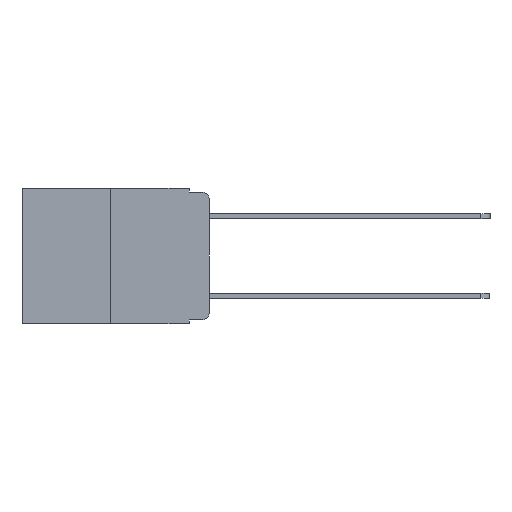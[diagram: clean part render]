
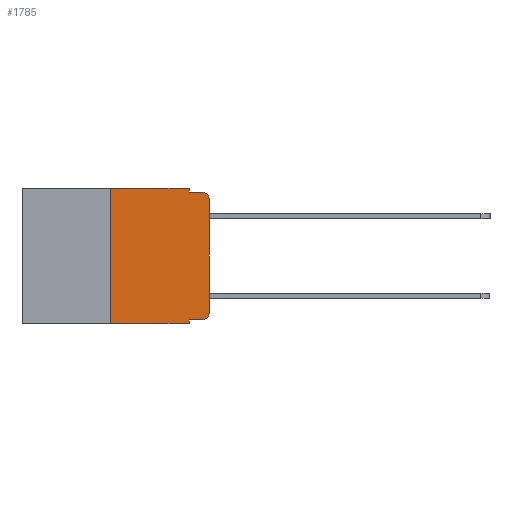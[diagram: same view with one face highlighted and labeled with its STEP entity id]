
A CAD part, left-side view. The second image highlights one B-rep face of the part: STEP entity #1785.
In plain terms, the highlighted planar face has unit normal (-1, 0, 0).
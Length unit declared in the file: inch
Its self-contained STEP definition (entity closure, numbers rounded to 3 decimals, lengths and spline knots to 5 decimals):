
#318 = LINE ( 'NONE', #8978, #4786 ) ;
#634 = DIRECTION ( 'NONE',  ( 0., 0., -1. ) ) ;
#671 = EDGE_CURVE ( 'NONE', #1986, #4047, #6278, .T. ) ;
#700 = ORIENTED_EDGE ( 'NONE', *, *, #8965, .T. ) ;
#863 = ORIENTED_EDGE ( 'NONE', *, *, #8610, .F. ) ;
#1166 = DIRECTION ( 'NONE',  ( 0., 0., 1. ) ) ;
#1209 = ORIENTED_EDGE ( 'NONE', *, *, #671, .T. ) ;
#1456 = ORIENTED_EDGE ( 'NONE', *, *, #9752, .T. ) ;
#1615 = ORIENTED_EDGE ( 'NONE', *, *, #4292, .F. ) ;
#1785 = ADVANCED_FACE ( 'NONE', ( #6901 ), #2590, .F. ) ;
#1864 = DIRECTION ( 'NONE',  ( 0., 0., -1. ) ) ;
#1952 = EDGE_CURVE ( 'NONE', #1986, #9415, #2936, .T. ) ;
#1986 = VERTEX_POINT ( 'NONE', #9089 ) ;
#2012 = VECTOR ( 'NONE', #9869, 39.37008 ) ;
#2094 = CARTESIAN_POINT ( 'NONE',  ( 0., 0.051, 0. ) ) ;
#2406 = CARTESIAN_POINT ( 'NONE',  ( 0., 0.051, 0. ) ) ;
#2559 = EDGE_CURVE ( 'NONE', #4123, #5530, #9926, .T. ) ;
#2590 = PLANE ( 'NONE',  #7639 ) ;
#2789 = CARTESIAN_POINT ( 'NONE',  ( 0., 0.25, -0.343 ) ) ;
#2936 = LINE ( 'NONE', #2094, #5074 ) ;
#3040 = EDGE_LOOP ( 'NONE', ( #5571, #5815, #1615, #9763, #863, #8460, #700, #7127, #1209, #1456 ) ) ;
#3163 = EDGE_CURVE ( 'NONE', #5752, #3700, #9809, .T. ) ;
#3416 = VERTEX_POINT ( 'NONE', #9243 ) ;
#3487 = DIRECTION ( 'NONE',  ( 0., -1., 0. ) ) ;
#3700 = VERTEX_POINT ( 'NONE', #3841 ) ;
#3841 = CARTESIAN_POINT ( 'NONE',  ( 0., 0.051, -0.01 ) ) ;
#4047 = VERTEX_POINT ( 'NONE', #9919 ) ;
#4123 = VERTEX_POINT ( 'NONE', #2789 ) ;
#4292 = EDGE_CURVE ( 'NONE', #3700, #6510, #7077, .T. ) ;
#4492 = CARTESIAN_POINT ( 'NONE',  ( 0., 0.051, 0. ) ) ;
#4639 = DIRECTION ( 'NONE',  ( -1., 0., 0. ) ) ;
#4687 = CARTESIAN_POINT ( 'NONE',  ( 0., 0.473, -0.343 ) ) ;
#4701 = VECTOR ( 'NONE', #5341, 39.37008 ) ;
#4786 = VECTOR ( 'NONE', #1166, 39.37008 ) ;
#5074 = VECTOR ( 'NONE', #1864, 39.37008 ) ;
#5341 = DIRECTION ( 'NONE',  ( 0., 0., 1. ) ) ;
#5471 = CARTESIAN_POINT ( 'NONE',  ( 0., 0.25, 0. ) ) ;
#5530 = VERTEX_POINT ( 'NONE', #6187 ) ;
#5571 = ORIENTED_EDGE ( 'NONE', *, *, #6310, .T. ) ;
#5752 = VERTEX_POINT ( 'NONE', #2406 ) ;
#5759 = DIRECTION ( 'NONE',  ( 1., 0., 0. ) ) ;
#5780 = DIRECTION ( 'NONE',  ( -1., 0., 0. ) ) ;
#5815 = ORIENTED_EDGE ( 'NONE', *, *, #5833, .T. ) ;
#5833 = EDGE_CURVE ( 'NONE', #3416, #6510, #7045, .T. ) ;
#5848 = DIRECTION ( 'NONE',  ( 0., 0., -1. ) ) ;
#6154 = DIRECTION ( 'NONE',  ( 0., -1., 0. ) ) ;
#6187 = CARTESIAN_POINT ( 'NONE',  ( 0., 0.25, 0. ) ) ;
#6218 = AXIS2_PLACEMENT_3D ( 'NONE', #8957, #4639, #9632 ) ;
#6278 = LINE ( 'NONE', #9307, #9760 ) ;
#6310 = EDGE_CURVE ( 'NONE', #8606, #3416, #318, .T. ) ;
#6385 = LINE ( 'NONE', #7255, #7821 ) ;
#6510 = VERTEX_POINT ( 'NONE', #7057 ) ;
#6552 = CARTESIAN_POINT ( 'NONE',  ( 0., 0., -0.313 ) ) ;
#6607 = CARTESIAN_POINT ( 'NONE',  ( 0., 0.051, -0.343 ) ) ;
#6901 = FACE_OUTER_BOUND ( 'NONE', #3040, .T. ) ;
#6953 = CARTESIAN_POINT ( 'NONE',  ( 0., 0.473, 0. ) ) ;
#7045 = CIRCLE ( 'NONE', #9470, 0.02 ) ;
#7057 = CARTESIAN_POINT ( 'NONE',  ( 0., 0.02, -0.01 ) ) ;
#7077 = LINE ( 'NONE', #9620, #8955 ) ;
#7127 = ORIENTED_EDGE ( 'NONE', *, *, #1952, .F. ) ;
#7133 = CIRCLE ( 'NONE', #6218, 0.02 ) ;
#7255 = CARTESIAN_POINT ( 'NONE',  ( 0., 0.473, 0. ) ) ;
#7639 = AXIS2_PLACEMENT_3D ( 'NONE', #6953, #5759, #5848 ) ;
#7821 = VECTOR ( 'NONE', #3487, 39.37008 ) ;
#8298 = DIRECTION ( 'NONE',  ( 0., -1., 0. ) ) ;
#8460 = ORIENTED_EDGE ( 'NONE', *, *, #2559, .F. ) ;
#8467 = VECTOR ( 'NONE', #8298, 39.37008 ) ;
#8606 = VERTEX_POINT ( 'NONE', #6552 ) ;
#8610 = EDGE_CURVE ( 'NONE', #5530, #5752, #6385, .T. ) ;
#8690 = LINE ( 'NONE', #4687, #8467 ) ;
#8955 = VECTOR ( 'NONE', #6154, 39.37008 ) ;
#8957 = CARTESIAN_POINT ( 'NONE',  ( 0., 0.02, -0.313 ) ) ;
#8965 = EDGE_CURVE ( 'NONE', #4123, #9415, #8690, .T. ) ;
#8978 = CARTESIAN_POINT ( 'NONE',  ( 0., 0., 0. ) ) ;
#9089 = CARTESIAN_POINT ( 'NONE',  ( 0., 0.051, -0.333 ) ) ;
#9208 = DIRECTION ( 'NONE',  ( 0., -1., 0. ) ) ;
#9243 = CARTESIAN_POINT ( 'NONE',  ( 0., 0., -0.03 ) ) ;
#9307 = CARTESIAN_POINT ( 'NONE',  ( 0., 0.051, -0.333 ) ) ;
#9415 = VERTEX_POINT ( 'NONE', #6607 ) ;
#9470 = AXIS2_PLACEMENT_3D ( 'NONE', #9940, #5780, #634 ) ;
#9620 = CARTESIAN_POINT ( 'NONE',  ( 0., 0.051, -0.01 ) ) ;
#9632 = DIRECTION ( 'NONE',  ( 0., 0., -1. ) ) ;
#9752 = EDGE_CURVE ( 'NONE', #4047, #8606, #7133, .T. ) ;
#9760 = VECTOR ( 'NONE', #9208, 39.37008 ) ;
#9763 = ORIENTED_EDGE ( 'NONE', *, *, #3163, .F. ) ;
#9809 = LINE ( 'NONE', #4492, #2012 ) ;
#9869 = DIRECTION ( 'NONE',  ( 0., 0., -1. ) ) ;
#9919 = CARTESIAN_POINT ( 'NONE',  ( 0., 0.02, -0.333 ) ) ;
#9926 = LINE ( 'NONE', #5471, #4701 ) ;
#9940 = CARTESIAN_POINT ( 'NONE',  ( 0., 0.02, -0.03 ) ) ;
